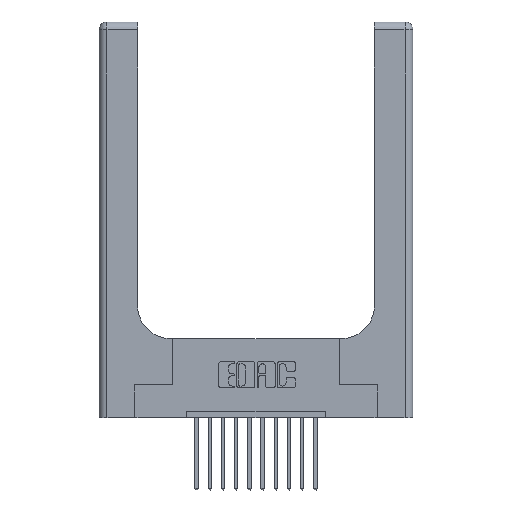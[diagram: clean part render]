
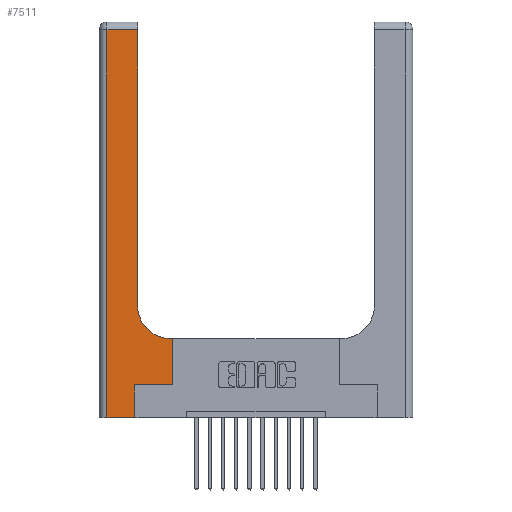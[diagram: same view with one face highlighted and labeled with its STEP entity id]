
A CAD part, top view. The second image highlights one B-rep face of the part: STEP entity #7511.
In plain terms, the highlighted planar face has unit normal (0, 0, 1).
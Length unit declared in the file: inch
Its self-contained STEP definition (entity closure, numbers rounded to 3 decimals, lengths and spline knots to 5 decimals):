
#212 = ORIENTED_EDGE ( 'NONE', *, *, #10947, .T. ) ;
#527 = VERTEX_POINT ( 'NONE', #2812 ) ;
#647 = LINE ( 'NONE', #1029, #13414 ) ;
#686 = DIRECTION ( 'NONE',  ( -1., 0., 0. ) ) ;
#1029 = CARTESIAN_POINT ( 'NONE',  ( 0.269, 0.25, 0.37 ) ) ;
#1088 = DIRECTION ( 'NONE',  ( 0., 1., 0. ) ) ;
#1443 = LINE ( 'NONE', #11280, #9865 ) ;
#1703 = CARTESIAN_POINT ( 'NONE',  ( 0.269, 0.25, 0.37 ) ) ;
#2789 = VERTEX_POINT ( 'NONE', #6013 ) ;
#2812 = CARTESIAN_POINT ( 'NONE',  ( 0.5585, 0.6, 0.37 ) ) ;
#2929 = AXIS2_PLACEMENT_3D ( 'NONE', #14032, #4947, #3564 ) ;
#3140 = LINE ( 'NONE', #12438, #13628 ) ;
#3246 = VECTOR ( 'NONE', #1088, 39.37008 ) ;
#3295 = VECTOR ( 'NONE', #16190, 39.37008 ) ;
#3318 = VERTEX_POINT ( 'NONE', #8416 ) ;
#3343 = ORIENTED_EDGE ( 'NONE', *, *, #6601, .T. ) ;
#3424 = ORIENTED_EDGE ( 'NONE', *, *, #15673, .T. ) ;
#3471 = LINE ( 'NONE', #12137, #13995 ) ;
#3474 = DIRECTION ( 'NONE',  ( 0., 0., -1. ) ) ;
#3555 = CARTESIAN_POINT ( 'NONE',  ( 0.269, 0., 0.37 ) ) ;
#3564 = DIRECTION ( 'NONE',  ( -1., 0., 0. ) ) ;
#3875 = DIRECTION ( 'NONE',  ( 0., -1., 0. ) ) ;
#4609 = VERTEX_POINT ( 'NONE', #6850 ) ;
#4696 = DIRECTION ( 'NONE',  ( 0., 1., 0. ) ) ;
#4699 = EDGE_CURVE ( 'NONE', #527, #2789, #1443, .T. ) ;
#4947 = DIRECTION ( 'NONE',  ( 0., 0., -1. ) ) ;
#5408 = LINE ( 'NONE', #15845, #15890 ) ;
#5527 = CARTESIAN_POINT ( 'NONE',  ( 0.2915, 2.94, 0.37 ) ) ;
#5646 = VERTEX_POINT ( 'NONE', #5527 ) ;
#5743 = LINE ( 'NONE', #8957, #3246 ) ;
#6013 = CARTESIAN_POINT ( 'NONE',  ( 0.5415, 0.6, 0.37 ) ) ;
#6082 = ORIENTED_EDGE ( 'NONE', *, *, #10852, .T. ) ;
#6601 = EDGE_CURVE ( 'NONE', #2789, #15801, #9598, .T. ) ;
#6666 = EDGE_LOOP ( 'NONE', ( #212, #6082, #10363, #7073, #13119, #14330, #3424, #8902, #3343 ) ) ;
#6850 = CARTESIAN_POINT ( 'NONE',  ( 0.06, 2.94, 0.37 ) ) ;
#7073 = ORIENTED_EDGE ( 'NONE', *, *, #15122, .T. ) ;
#7511 = ADVANCED_FACE ( 'NONE', ( #10187 ), #14211, .F. ) ;
#7516 = DIRECTION ( 'NONE',  ( -1., 0., 0. ) ) ;
#8416 = CARTESIAN_POINT ( 'NONE',  ( 0.06, 0., 0.37 ) ) ;
#8572 = CARTESIAN_POINT ( 'NONE',  ( 0.5585, 0.25, 0.37 ) ) ;
#8770 = CARTESIAN_POINT ( 'NONE',  ( 0.5415, 0.85, 0.37 ) ) ;
#8902 = ORIENTED_EDGE ( 'NONE', *, *, #4699, .T. ) ;
#8957 = CARTESIAN_POINT ( 'NONE',  ( 0.2915, 3., 0.37 ) ) ;
#9598 = CIRCLE ( 'NONE', #12233, 0.25 ) ;
#9611 = VERTEX_POINT ( 'NONE', #1703 ) ;
#9619 = DIRECTION ( 'NONE',  ( 0., 1., 0. ) ) ;
#9865 = VECTOR ( 'NONE', #7516, 39.37008 ) ;
#10049 = CARTESIAN_POINT ( 'NONE',  ( 0., 2.94, 0.37 ) ) ;
#10187 = FACE_OUTER_BOUND ( 'NONE', #6666, .T. ) ;
#10363 = ORIENTED_EDGE ( 'NONE', *, *, #14063, .T. ) ;
#10852 = EDGE_CURVE ( 'NONE', #5646, #4609, #16202, .T. ) ;
#10903 = VERTEX_POINT ( 'NONE', #8572 ) ;
#10947 = EDGE_CURVE ( 'NONE', #15801, #5646, #5743, .T. ) ;
#11112 = CARTESIAN_POINT ( 'NONE',  ( 0., 0., 0.37 ) ) ;
#11280 = CARTESIAN_POINT ( 'NONE',  ( 0.2915, 0.6, 0.37 ) ) ;
#11608 = CARTESIAN_POINT ( 'NONE',  ( 0.2915, 0.85, 0.37 ) ) ;
#11670 = DIRECTION ( 'NONE',  ( 1., 0., 0. ) ) ;
#11929 = LINE ( 'NONE', #11112, #3295 ) ;
#12137 = CARTESIAN_POINT ( 'NONE',  ( 0.5585, 0.25, 0.37 ) ) ;
#12233 = AXIS2_PLACEMENT_3D ( 'NONE', #8770, #3474, #12669 ) ;
#12438 = CARTESIAN_POINT ( 'NONE',  ( 0.269, 0., 0.37 ) ) ;
#12669 = DIRECTION ( 'NONE',  ( 1., 0., 0. ) ) ;
#13119 = ORIENTED_EDGE ( 'NONE', *, *, #13880, .T. ) ;
#13414 = VECTOR ( 'NONE', #11670, 39.37008 ) ;
#13628 = VECTOR ( 'NONE', #4696, 39.37008 ) ;
#13880 = EDGE_CURVE ( 'NONE', #14642, #9611, #3140, .T. ) ;
#13995 = VECTOR ( 'NONE', #9619, 39.37008 ) ;
#14032 = CARTESIAN_POINT ( 'NONE',  ( 0., 3., 0.37 ) ) ;
#14063 = EDGE_CURVE ( 'NONE', #4609, #3318, #5408, .T. ) ;
#14211 = PLANE ( 'NONE',  #2929 ) ;
#14305 = EDGE_CURVE ( 'NONE', #9611, #10903, #647, .T. ) ;
#14330 = ORIENTED_EDGE ( 'NONE', *, *, #14305, .T. ) ;
#14585 = VECTOR ( 'NONE', #686, 39.37008 ) ;
#14642 = VERTEX_POINT ( 'NONE', #3555 ) ;
#15122 = EDGE_CURVE ( 'NONE', #3318, #14642, #11929, .T. ) ;
#15673 = EDGE_CURVE ( 'NONE', #10903, #527, #3471, .T. ) ;
#15801 = VERTEX_POINT ( 'NONE', #11608 ) ;
#15845 = CARTESIAN_POINT ( 'NONE',  ( 0.06, 3., 0.37 ) ) ;
#15890 = VECTOR ( 'NONE', #3875, 39.37008 ) ;
#16190 = DIRECTION ( 'NONE',  ( 1., 0., 0. ) ) ;
#16202 = LINE ( 'NONE', #10049, #14585 ) ;
